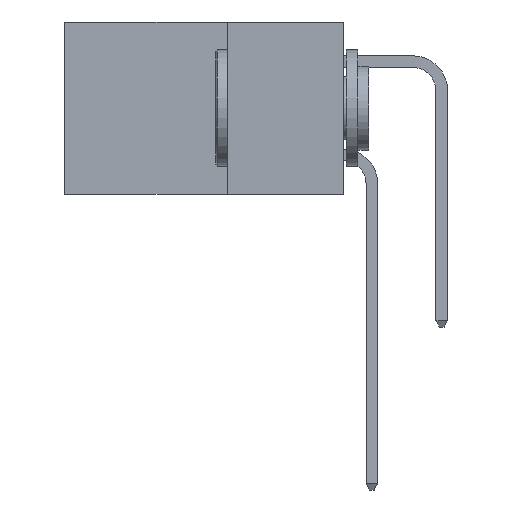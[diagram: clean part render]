
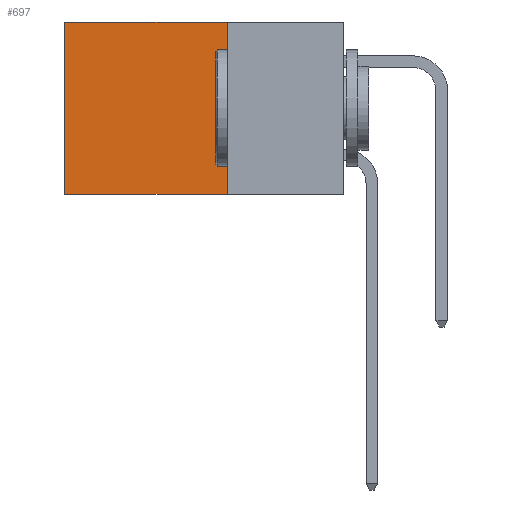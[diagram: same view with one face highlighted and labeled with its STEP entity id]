
A CAD part, left-side view. The second image highlights one B-rep face of the part: STEP entity #697.
In plain terms, the highlighted planar face has unit normal (-1, 0, 0).
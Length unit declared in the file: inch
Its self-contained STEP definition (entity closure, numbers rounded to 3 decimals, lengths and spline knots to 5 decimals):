
#697 = ADVANCED_FACE ( 'NONE', ( #11658 ), #9409, .F. ) ;
#715 = EDGE_CURVE ( 'NONE', #3508, #14704, #11241, .T. ) ;
#1595 = VERTEX_POINT ( 'NONE', #7439 ) ;
#3118 = ORIENTED_EDGE ( 'NONE', *, *, #715, .T. ) ;
#3447 = LINE ( 'NONE', #15272, #16953 ) ;
#3508 = VERTEX_POINT ( 'NONE', #6670 ) ;
#4071 = ORIENTED_EDGE ( 'NONE', *, *, #7453, .F. ) ;
#4482 = VECTOR ( 'NONE', #9804, 39.37008 ) ;
#4602 = VECTOR ( 'NONE', #5397, 39.37008 ) ;
#5000 = CARTESIAN_POINT ( 'NONE',  ( 0.2615, 0.25, -0.37 ) ) ;
#5009 = LINE ( 'NONE', #5564, #4602 ) ;
#5159 = VECTOR ( 'NONE', #9515, 39.37008 ) ;
#5397 = DIRECTION ( 'NONE',  ( 0., 1., 0. ) ) ;
#5564 = CARTESIAN_POINT ( 'NONE',  ( 0.2615, 0.25, -0.37 ) ) ;
#6670 = CARTESIAN_POINT ( 'NONE',  ( 0.2615, 0.25, 0. ) ) ;
#7198 = AXIS2_PLACEMENT_3D ( 'NONE', #7562, #14256, #14190 ) ;
#7439 = CARTESIAN_POINT ( 'NONE',  ( 0.2615, 0.6, -0.37 ) ) ;
#7453 = EDGE_CURVE ( 'NONE', #3508, #15056, #3447, .T. ) ;
#7562 = CARTESIAN_POINT ( 'NONE',  ( 0.2615, 0.25, -0.37 ) ) ;
#7710 = CARTESIAN_POINT ( 'NONE',  ( 0.2615, 0.6, 0. ) ) ;
#9013 = ORIENTED_EDGE ( 'NONE', *, *, #14164, .T. ) ;
#9172 = CARTESIAN_POINT ( 'NONE',  ( 0.2615, 0.6, -0.37 ) ) ;
#9301 = CARTESIAN_POINT ( 'NONE',  ( 0.2615, 0.25, 0. ) ) ;
#9409 = PLANE ( 'NONE',  #7198 ) ;
#9515 = DIRECTION ( 'NONE',  ( 0., 0., -1. ) ) ;
#9804 = DIRECTION ( 'NONE',  ( 0., 1., 0. ) ) ;
#9983 = EDGE_LOOP ( 'NONE', ( #9013, #10104, #4071, #3118 ) ) ;
#10104 = ORIENTED_EDGE ( 'NONE', *, *, #10787, .F. ) ;
#10787 = EDGE_CURVE ( 'NONE', #15056, #1595, #5009, .T. ) ;
#11241 = LINE ( 'NONE', #9301, #4482 ) ;
#11658 = FACE_OUTER_BOUND ( 'NONE', #9983, .T. ) ;
#12333 = LINE ( 'NONE', #9172, #5159 ) ;
#14164 = EDGE_CURVE ( 'NONE', #14704, #1595, #12333, .T. ) ;
#14190 = DIRECTION ( 'NONE',  ( 0., 0., -1. ) ) ;
#14256 = DIRECTION ( 'NONE',  ( 1., 0., 0. ) ) ;
#14704 = VERTEX_POINT ( 'NONE', #7710 ) ;
#15056 = VERTEX_POINT ( 'NONE', #5000 ) ;
#15238 = DIRECTION ( 'NONE',  ( 0., 0., -1. ) ) ;
#15272 = CARTESIAN_POINT ( 'NONE',  ( 0.2615, 0.25, -0.37 ) ) ;
#16953 = VECTOR ( 'NONE', #15238, 39.37008 ) ;
